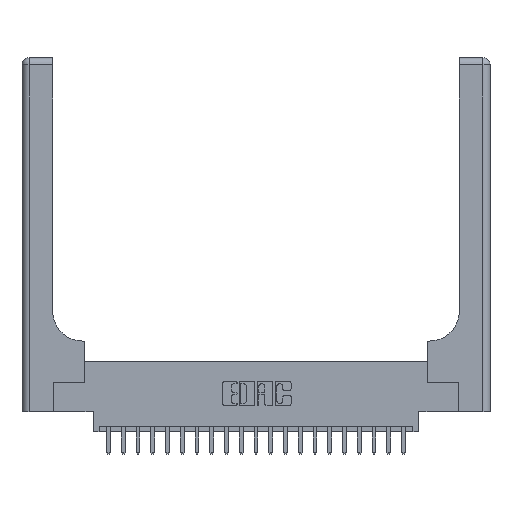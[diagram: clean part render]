
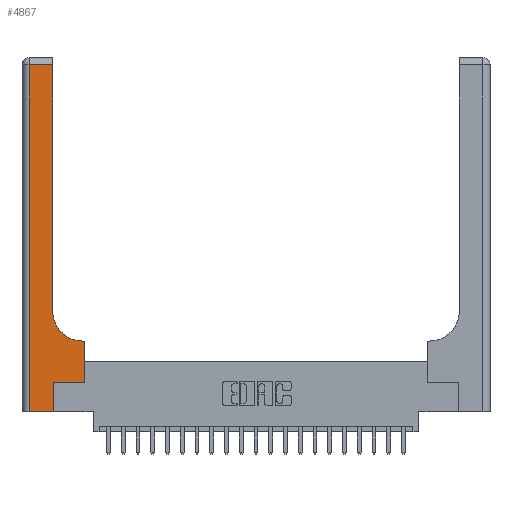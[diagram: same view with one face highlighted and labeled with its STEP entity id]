
A CAD part, top view. The second image highlights one B-rep face of the part: STEP entity #4867.
In plain terms, the highlighted planar face has unit normal (0, 0, 1).
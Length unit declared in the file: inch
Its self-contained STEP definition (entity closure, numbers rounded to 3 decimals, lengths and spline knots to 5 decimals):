
#102 = DIRECTION ( 'NONE',  ( 0., 0., -1. ) ) ;
#543 = AXIS2_PLACEMENT_3D ( 'NONE', #9416, #4189, #12595 ) ;
#795 = AXIS2_PLACEMENT_3D ( 'NONE', #4951, #102, #11871 ) ;
#1222 = CARTESIAN_POINT ( 'NONE',  ( 0.528, 0.25, 0.37 ) ) ;
#1271 = LINE ( 'NONE', #8280, #4989 ) ;
#1299 = VERTEX_POINT ( 'NONE', #16147 ) ;
#1315 = CARTESIAN_POINT ( 'NONE',  ( 0.265, 0.25, 0.37 ) ) ;
#1908 = CARTESIAN_POINT ( 'NONE',  ( 0.26, 0.85, 0.37 ) ) ;
#1931 = LINE ( 'NONE', #21013, #8745 ) ;
#2342 = DIRECTION ( 'NONE',  ( 1., 0., 0. ) ) ;
#2559 = LINE ( 'NONE', #15967, #8693 ) ;
#2684 = DIRECTION ( 'NONE',  ( 0., 1., 0. ) ) ;
#3327 = VERTEX_POINT ( 'NONE', #16456 ) ;
#3829 = EDGE_CURVE ( 'NONE', #21201, #13465, #9461, .T. ) ;
#3931 = VECTOR ( 'NONE', #5846, 39.37008 ) ;
#3985 = DIRECTION ( 'NONE',  ( 1., 0., 0. ) ) ;
#4169 = CARTESIAN_POINT ( 'NONE',  ( 0.528, 0.6, 0.37 ) ) ;
#4189 = DIRECTION ( 'NONE',  ( 0., 0., -1. ) ) ;
#4292 = ORIENTED_EDGE ( 'NONE', *, *, #6539, .T. ) ;
#4831 = CARTESIAN_POINT ( 'NONE',  ( 0.265, 0., 0.37 ) ) ;
#4867 = ADVANCED_FACE ( 'NONE', ( #12833 ), #11004, .F. ) ;
#4951 = CARTESIAN_POINT ( 'NONE',  ( 0.51, 0.85, 0.37 ) ) ;
#4989 = VECTOR ( 'NONE', #15341, 39.37008 ) ;
#5209 = VERTEX_POINT ( 'NONE', #9905 ) ;
#5593 = ORIENTED_EDGE ( 'NONE', *, *, #21305, .T. ) ;
#5692 = VERTEX_POINT ( 'NONE', #9327 ) ;
#5846 = DIRECTION ( 'NONE',  ( 0., -1., 0. ) ) ;
#5935 = VERTEX_POINT ( 'NONE', #19047 ) ;
#6155 = VECTOR ( 'NONE', #3985, 39.37008 ) ;
#6539 = EDGE_CURVE ( 'NONE', #5692, #5209, #7664, .T. ) ;
#6915 = ORIENTED_EDGE ( 'NONE', *, *, #10025, .T. ) ;
#7106 = EDGE_CURVE ( 'NONE', #1299, #5692, #1271, .T. ) ;
#7254 = DIRECTION ( 'NONE',  ( 0., 1., 0. ) ) ;
#7277 = CIRCLE ( 'NONE', #795, 0.25 ) ;
#7324 = CARTESIAN_POINT ( 'NONE',  ( 0.51, 0.6, 0.37 ) ) ;
#7664 = LINE ( 'NONE', #7987, #3931 ) ;
#7977 = CARTESIAN_POINT ( 'NONE',  ( 0.26, 0.6, 0.37 ) ) ;
#7987 = CARTESIAN_POINT ( 'NONE',  ( 0.06, 3., 0.37 ) ) ;
#8101 = VECTOR ( 'NONE', #16830, 39.37008 ) ;
#8280 = CARTESIAN_POINT ( 'NONE',  ( 0., 2.94, 0.37 ) ) ;
#8693 = VECTOR ( 'NONE', #2342, 39.37008 ) ;
#8745 = VECTOR ( 'NONE', #7254, 39.37008 ) ;
#9327 = CARTESIAN_POINT ( 'NONE',  ( 0.06, 2.94, 0.37 ) ) ;
#9416 = CARTESIAN_POINT ( 'NONE',  ( 0., 3., 0.37 ) ) ;
#9461 = LINE ( 'NONE', #7977, #8101 ) ;
#9612 = EDGE_CURVE ( 'NONE', #5209, #5935, #19217, .T. ) ;
#9905 = CARTESIAN_POINT ( 'NONE',  ( 0.06, 0., 0.37 ) ) ;
#10025 = EDGE_CURVE ( 'NONE', #13971, #3327, #2559, .T. ) ;
#11004 = PLANE ( 'NONE',  #543 ) ;
#11229 = EDGE_CURVE ( 'NONE', #18110, #1299, #1931, .T. ) ;
#11754 = DIRECTION ( 'NONE',  ( 0., 1., 0. ) ) ;
#11871 = DIRECTION ( 'NONE',  ( 1., 0., 0. ) ) ;
#12595 = DIRECTION ( 'NONE',  ( -1., 0., 0. ) ) ;
#12833 = FACE_OUTER_BOUND ( 'NONE', #14883, .T. ) ;
#13465 = VERTEX_POINT ( 'NONE', #7324 ) ;
#13971 = VERTEX_POINT ( 'NONE', #1315 ) ;
#14341 = CARTESIAN_POINT ( 'NONE',  ( 0., 0., 0.37 ) ) ;
#14557 = ORIENTED_EDGE ( 'NONE', *, *, #7106, .T. ) ;
#14861 = LINE ( 'NONE', #1222, #15623 ) ;
#14883 = EDGE_LOOP ( 'NONE', ( #22259, #14557, #4292, #22276, #22186, #6915, #5593, #19780, #15471 ) ) ;
#15180 = VECTOR ( 'NONE', #11754, 39.37008 ) ;
#15341 = DIRECTION ( 'NONE',  ( -1., 0., 0. ) ) ;
#15471 = ORIENTED_EDGE ( 'NONE', *, *, #21458, .T. ) ;
#15623 = VECTOR ( 'NONE', #2684, 39.37008 ) ;
#15967 = CARTESIAN_POINT ( 'NONE',  ( 0.265, 0.25, 0.37 ) ) ;
#16147 = CARTESIAN_POINT ( 'NONE',  ( 0.26, 2.94, 0.37 ) ) ;
#16456 = CARTESIAN_POINT ( 'NONE',  ( 0.528, 0.25, 0.37 ) ) ;
#16830 = DIRECTION ( 'NONE',  ( -1., 0., 0. ) ) ;
#17042 = EDGE_CURVE ( 'NONE', #5935, #13971, #20865, .T. ) ;
#18110 = VERTEX_POINT ( 'NONE', #1908 ) ;
#19047 = CARTESIAN_POINT ( 'NONE',  ( 0.265, 0., 0.37 ) ) ;
#19217 = LINE ( 'NONE', #14341, #6155 ) ;
#19780 = ORIENTED_EDGE ( 'NONE', *, *, #3829, .T. ) ;
#20865 = LINE ( 'NONE', #4831, #15180 ) ;
#21013 = CARTESIAN_POINT ( 'NONE',  ( 0.26, 3., 0.37 ) ) ;
#21201 = VERTEX_POINT ( 'NONE', #4169 ) ;
#21305 = EDGE_CURVE ( 'NONE', #3327, #21201, #14861, .T. ) ;
#21458 = EDGE_CURVE ( 'NONE', #13465, #18110, #7277, .T. ) ;
#22186 = ORIENTED_EDGE ( 'NONE', *, *, #17042, .T. ) ;
#22259 = ORIENTED_EDGE ( 'NONE', *, *, #11229, .T. ) ;
#22276 = ORIENTED_EDGE ( 'NONE', *, *, #9612, .T. ) ;
